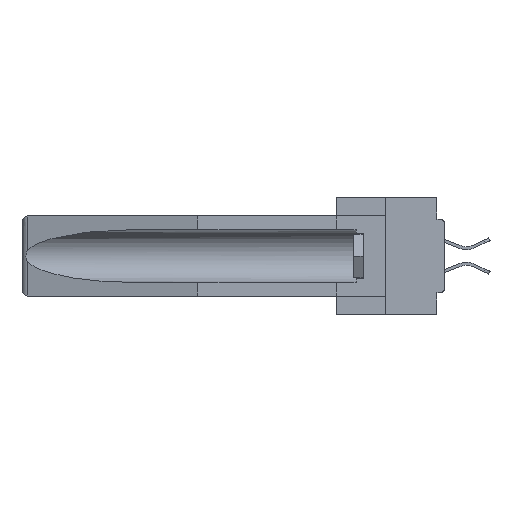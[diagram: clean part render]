
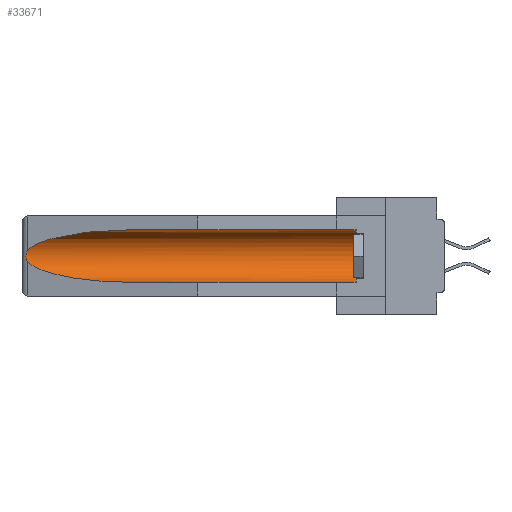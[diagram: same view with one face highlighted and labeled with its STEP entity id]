
A CAD part, left-side view. The second image highlights one B-rep face of the part: STEP entity #33671.
In plain terms, the highlighted cylindrical face has radius 2.857 mm (diameter 5.715 mm), a partial arc.
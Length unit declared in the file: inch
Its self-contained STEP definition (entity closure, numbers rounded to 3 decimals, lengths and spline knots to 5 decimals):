
#828 =( BOUNDED_CURVE ( )  B_SPLINE_CURVE ( 3, ( #38498, #18630, #35114, #8120 ),
 .UNSPECIFIED., .F., .T. ) 
 B_SPLINE_CURVE_WITH_KNOTS ( ( 4, 4 ),
 ( 4.71239, 6.08839 ),
 .UNSPECIFIED. ) 
 CURVE ( )  GEOMETRIC_REPRESENTATION_ITEM ( )  RATIONAL_B_SPLINE_CURVE ( ( 1., 0.848, 0.848, 1. ) ) 
 REPRESENTATION_ITEM ( '' )  );
#2423 = CARTESIAN_POINT ( 'NONE',  ( 0.25451, 1.48313, -0.24835 ) ) ;
#2498 = CARTESIAN_POINT ( 'NONE',  ( 0.26655, 1.53094, -0.18657 ) ) ;
#4845 = CARTESIAN_POINT ( 'NONE',  ( 0.26537, 1.52718, -0.14972 ) ) ;
#5287 = CARTESIAN_POINT ( 'NONE',  ( 0.2673, 1.5327, -0.16383 ) ) ;
#5869 = VERTEX_POINT ( 'NONE', #29700 ) ;
#6687 = CARTESIAN_POINT ( 'NONE',  ( 0.155, -0.30754, -0.284 ) ) ;
#7680 = EDGE_CURVE ( 'NONE', #5869, #25223, #39696, .T. ) ;
#8120 = CARTESIAN_POINT ( 'NONE',  ( 0.26537, 1.52718, -0.14972 ) ) ;
#8200 = ORIENTED_EDGE ( 'NONE', *, *, #7680, .T. ) ;
#9650 = VERTEX_POINT ( 'NONE', #36043 ) ;
#10149 = VECTOR ( 'NONE', #39829, 39.37008 ) ;
#12131 = EDGE_CURVE ( 'NONE', #9650, #37010, #16507, .T. ) ;
#12279 = LINE ( 'NONE', #6687, #10149 ) ;
#12281 = VERTEX_POINT ( 'NONE', #22477 ) ;
#13012 = CARTESIAN_POINT ( 'NONE',  ( 0.26537, 1.52718, -0.19328 ) ) ;
#13113 = EDGE_CURVE ( 'NONE', #12281, #9650, #31567, .T. ) ;
#13311 = VERTEX_POINT ( 'NONE', #38706 ) ;
#14342 = ORIENTED_EDGE ( 'NONE', *, *, #22494, .F. ) ;
#14936 = VECTOR ( 'NONE', #21368, 39.37008 ) ;
#16507 = LINE ( 'NONE', #37990, #14936 ) ;
#18576 = CARTESIAN_POINT ( 'NONE',  ( 0.26597, 1.52961, -0.15275 ) ) ;
#18630 = CARTESIAN_POINT ( 'NONE',  ( 0.21114, 1.30732, -0.059 ) ) ;
#18746 = ORIENTED_EDGE ( 'NONE', *, *, #13113, .T. ) ;
#21074 = DIRECTION ( 'NONE',  ( 0., 0., 1. ) ) ;
#21222 = CARTESIAN_POINT ( 'NONE',  ( 0.155, 0.126, -0.1715 ) ) ;
#21368 = DIRECTION ( 'NONE',  ( 0., 1., 0. ) ) ;
#21977 = CARTESIAN_POINT ( 'NONE',  ( 0.26654, 1.53092, -0.15636 ) ) ;
#22118 = CARTESIAN_POINT ( 'NONE',  ( 0.2675, 1.53308, -0.16763 ) ) ;
#22264 = ORIENTED_EDGE ( 'NONE', *, *, #41663, .T. ) ;
#22471 = CARTESIAN_POINT ( 'NONE',  ( 0.26537, 1.52718, -0.19328 ) ) ;
#22477 = CARTESIAN_POINT ( 'NONE',  ( 0.155, 0.126, -0.284 ) ) ;
#22494 = EDGE_CURVE ( 'NONE', #12281, #25223, #12279, .T. ) ;
#23096 = CARTESIAN_POINT ( 'NONE',  ( 0.2675, 1.53308, -0.17534 ) ) ;
#24212 = B_SPLINE_CURVE_WITH_KNOTS ( 'NONE', 3,
 ( #4845, #18576, #21977, #5287, #22118, #23096, #26502, #2498, #36205, #13012 ),
 .UNSPECIFIED., .F., .F.,
 ( 4, 2, 2, 2, 4 ),
 ( 0., 0.00029, 0.00058, 0.00087, 0.00117 ),
 .UNSPECIFIED. ) ;
#24519 = ORIENTED_EDGE ( 'NONE', *, *, #33206, .T. ) ;
#25223 = VERTEX_POINT ( 'NONE', #33064 ) ;
#25852 = CARTESIAN_POINT ( 'NONE',  ( 0.21114, 1.30732, -0.284 ) ) ;
#26502 = CARTESIAN_POINT ( 'NONE',  ( 0.2673, 1.53269, -0.17917 ) ) ;
#29194 = CARTESIAN_POINT ( 'NONE',  ( 0.155, 1.07973, -0.284 ) ) ;
#29700 = CARTESIAN_POINT ( 'NONE',  ( 0.26537, 1.52718, -0.19328 ) ) ;
#31567 = CIRCLE ( 'NONE', #41546, 0.1125 ) ;
#32413 = DIRECTION ( 'NONE',  ( 0., 1., 0. ) ) ;
#33029 = CYLINDRICAL_SURFACE ( 'NONE', #38859, 0.1125 ) ;
#33064 = CARTESIAN_POINT ( 'NONE',  ( 0.155, 1.07973, -0.284 ) ) ;
#33206 = EDGE_CURVE ( 'NONE', #13311, #5869, #24212, .T. ) ;
#33671 = ADVANCED_FACE ( 'NONE', ( #38256 ), #33029, .F. ) ;
#34331 = DIRECTION ( 'NONE',  ( 0., -1., 0. ) ) ;
#35114 = CARTESIAN_POINT ( 'NONE',  ( 0.25451, 1.48313, -0.09465 ) ) ;
#35447 = CARTESIAN_POINT ( 'NONE',  ( 0.155, -0.30754, -0.1715 ) ) ;
#36043 = CARTESIAN_POINT ( 'NONE',  ( 0.155, 0.126, -0.059 ) ) ;
#36205 = CARTESIAN_POINT ( 'NONE',  ( 0.26597, 1.5296, -0.19026 ) ) ;
#37010 = VERTEX_POINT ( 'NONE', #40708 ) ;
#37697 = EDGE_LOOP ( 'NONE', ( #22264, #24519, #8200, #14342, #18746, #42045 ) ) ;
#37990 = CARTESIAN_POINT ( 'NONE',  ( 0.155, -0.30754, -0.059 ) ) ;
#38256 = FACE_OUTER_BOUND ( 'NONE', #37697, .T. ) ;
#38498 = CARTESIAN_POINT ( 'NONE',  ( 0.155, 1.07973, -0.059 ) ) ;
#38706 = CARTESIAN_POINT ( 'NONE',  ( 0.26537, 1.52718, -0.14972 ) ) ;
#38832 = DIRECTION ( 'NONE',  ( 0., 0., 1. ) ) ;
#38859 = AXIS2_PLACEMENT_3D ( 'NONE', #35447, #32413, #38832 ) ;
#39696 =( BOUNDED_CURVE ( )  B_SPLINE_CURVE ( 3, ( #22471, #2423, #25852, #29194 ),
 .UNSPECIFIED., .F., .F. ) 
 B_SPLINE_CURVE_WITH_KNOTS ( ( 4, 4 ),
 ( 0.1948, 1.5708 ),
 .UNSPECIFIED. ) 
 CURVE ( )  GEOMETRIC_REPRESENTATION_ITEM ( )  RATIONAL_B_SPLINE_CURVE ( ( 1., 0.848, 0.848, 1. ) ) 
 REPRESENTATION_ITEM ( '' )  );
#39829 = DIRECTION ( 'NONE',  ( 0., 1., 0. ) ) ;
#40708 = CARTESIAN_POINT ( 'NONE',  ( 0.155, 1.07973, -0.059 ) ) ;
#41546 = AXIS2_PLACEMENT_3D ( 'NONE', #21222, #34331, #21074 ) ;
#41663 = EDGE_CURVE ( 'NONE', #37010, #13311, #828, .T. ) ;
#42045 = ORIENTED_EDGE ( 'NONE', *, *, #12131, .T. ) ;
